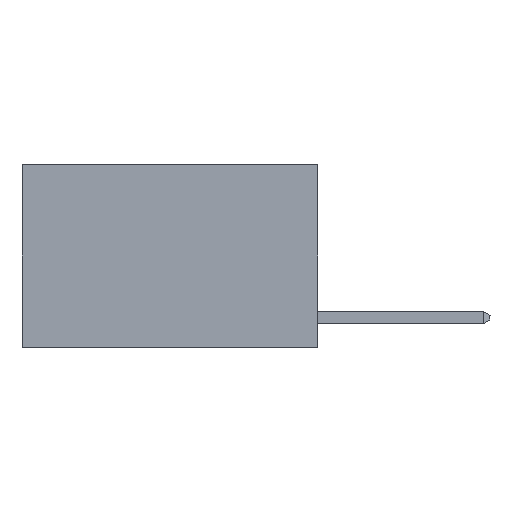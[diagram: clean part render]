
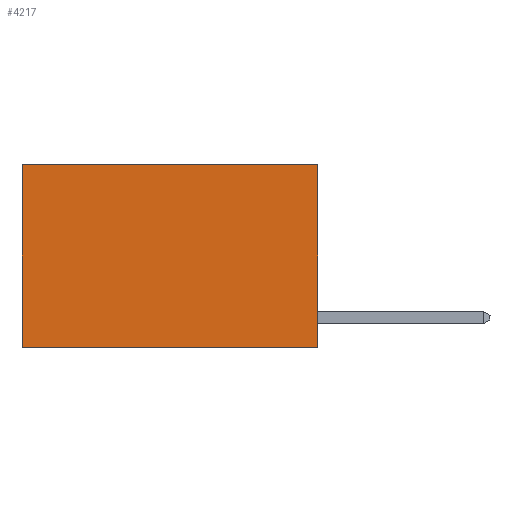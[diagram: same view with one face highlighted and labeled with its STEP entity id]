
A CAD part, left-side view. The second image highlights one B-rep face of the part: STEP entity #4217.
In plain terms, the highlighted planar face has unit normal (-1, 0, 0).
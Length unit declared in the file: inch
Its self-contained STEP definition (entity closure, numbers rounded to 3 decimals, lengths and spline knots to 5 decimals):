
#413 = ORIENTED_EDGE ( 'NONE', *, *, #6409, .F. ) ;
#531 = CARTESIAN_POINT ( 'NONE',  ( 0.2625, 0., 0. ) ) ;
#861 = EDGE_CURVE ( 'NONE', #8497, #8611, #12444, .T. ) ;
#947 = VECTOR ( 'NONE', #6107, 39.37008 ) ;
#983 = FACE_OUTER_BOUND ( 'NONE', #4301, .T. ) ;
#1543 = VECTOR ( 'NONE', #5926, 39.37008 ) ;
#1957 = CARTESIAN_POINT ( 'NONE',  ( 0.2625, 0., 0. ) ) ;
#2198 = LINE ( 'NONE', #10177, #1543 ) ;
#2379 = ORIENTED_EDGE ( 'NONE', *, *, #12030, .F. ) ;
#2527 = ORIENTED_EDGE ( 'NONE', *, *, #861, .T. ) ;
#3298 = CARTESIAN_POINT ( 'NONE',  ( 0.2625, 0.6, 0. ) ) ;
#3390 = CARTESIAN_POINT ( 'NONE',  ( 0.2625, 0.6, 0. ) ) ;
#3602 = DIRECTION ( 'NONE',  ( 0., 0., -1. ) ) ;
#4202 = CARTESIAN_POINT ( 'NONE',  ( 0.2625, 0., 0. ) ) ;
#4217 = ADVANCED_FACE ( 'NONE', ( #983 ), #9981, .F. ) ;
#4301 = EDGE_LOOP ( 'NONE', ( #2527, #2379, #413, #5531 ) ) ;
#4311 = VECTOR ( 'NONE', #6148, 39.37008 ) ;
#4855 = VERTEX_POINT ( 'NONE', #11395 ) ;
#5033 = LINE ( 'NONE', #1957, #947 ) ;
#5531 = ORIENTED_EDGE ( 'NONE', *, *, #9317, .T. ) ;
#5732 = CARTESIAN_POINT ( 'NONE',  ( 0.2625, 0., 0. ) ) ;
#5926 = DIRECTION ( 'NONE',  ( 0., 1., 0. ) ) ;
#6107 = DIRECTION ( 'NONE',  ( 0., 1., 0. ) ) ;
#6148 = DIRECTION ( 'NONE',  ( 0., 0., -1. ) ) ;
#6162 = AXIS2_PLACEMENT_3D ( 'NONE', #531, #10025, #3602 ) ;
#6409 = EDGE_CURVE ( 'NONE', #13450, #4855, #12745, .T. ) ;
#7401 = DIRECTION ( 'NONE',  ( 0., 0., -1. ) ) ;
#8497 = VERTEX_POINT ( 'NONE', #3298 ) ;
#8611 = VERTEX_POINT ( 'NONE', #9866 ) ;
#9317 = EDGE_CURVE ( 'NONE', #13450, #8497, #5033, .T. ) ;
#9866 = CARTESIAN_POINT ( 'NONE',  ( 0.2625, 0.6, -0.37 ) ) ;
#9981 = PLANE ( 'NONE',  #6162 ) ;
#10025 = DIRECTION ( 'NONE',  ( 1., 0., 0. ) ) ;
#10177 = CARTESIAN_POINT ( 'NONE',  ( 0.2625, 0., -0.37 ) ) ;
#11395 = CARTESIAN_POINT ( 'NONE',  ( 0.2625, 0., -0.37 ) ) ;
#11788 = VECTOR ( 'NONE', #7401, 39.37008 ) ;
#12030 = EDGE_CURVE ( 'NONE', #4855, #8611, #2198, .T. ) ;
#12444 = LINE ( 'NONE', #3390, #11788 ) ;
#12745 = LINE ( 'NONE', #4202, #4311 ) ;
#13450 = VERTEX_POINT ( 'NONE', #5732 ) ;
